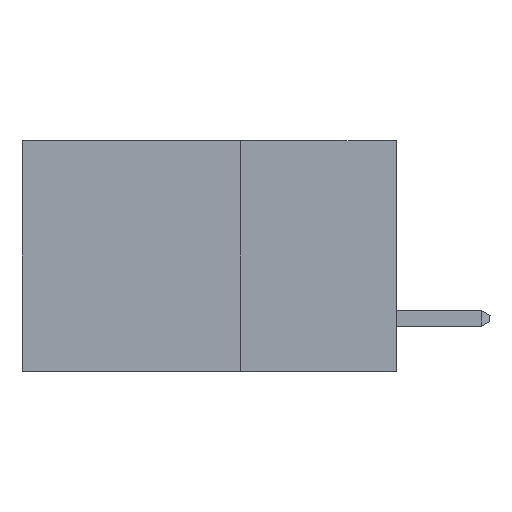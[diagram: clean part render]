
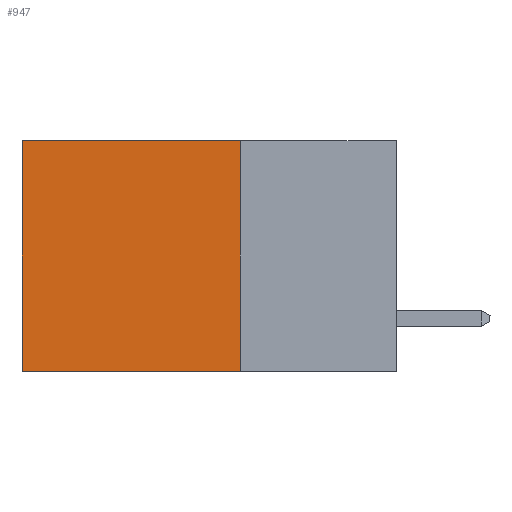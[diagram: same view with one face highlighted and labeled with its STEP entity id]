
A CAD part, left-side view. The second image highlights one B-rep face of the part: STEP entity #947.
In plain terms, the highlighted planar face has unit normal (-1, 0, 0).
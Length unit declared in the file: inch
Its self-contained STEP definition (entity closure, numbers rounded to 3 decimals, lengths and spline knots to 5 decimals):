
#130 = LINE ( 'NONE', #974, #3884 ) ;
#669 = EDGE_LOOP ( 'NONE', ( #11344, #8845, #17413, #20293 ) ) ;
#853 = FACE_OUTER_BOUND ( 'NONE', #669, .T. ) ;
#947 = ADVANCED_FACE ( 'NONE', ( #853 ), #6151, .F. ) ;
#974 = CARTESIAN_POINT ( 'NONE',  ( 0.298, 0.25, 0. ) ) ;
#1856 = VECTOR ( 'NONE', #12233, 39.37008 ) ;
#2338 = CARTESIAN_POINT ( 'NONE',  ( 0.298, 0.25, -0.37 ) ) ;
#2418 = CARTESIAN_POINT ( 'NONE',  ( 0.298, 0.25, 0. ) ) ;
#2761 = VERTEX_POINT ( 'NONE', #21534 ) ;
#3884 = VECTOR ( 'NONE', #17255, 39.37008 ) ;
#4468 = AXIS2_PLACEMENT_3D ( 'NONE', #13750, #15356, #18945 ) ;
#5245 = CARTESIAN_POINT ( 'NONE',  ( 0.298, 0.25, -0.37 ) ) ;
#6151 = PLANE ( 'NONE',  #4468 ) ;
#7152 = VECTOR ( 'NONE', #18747, 39.37008 ) ;
#8224 = LINE ( 'NONE', #8526, #1856 ) ;
#8526 = CARTESIAN_POINT ( 'NONE',  ( 0.298, 0.6, 0. ) ) ;
#8845 = ORIENTED_EDGE ( 'NONE', *, *, #14972, .F. ) ;
#11203 = LINE ( 'NONE', #18828, #7152 ) ;
#11344 = ORIENTED_EDGE ( 'NONE', *, *, #19478, .T. ) ;
#12024 = VERTEX_POINT ( 'NONE', #2418 ) ;
#12233 = DIRECTION ( 'NONE',  ( 0., 0., -1. ) ) ;
#12912 = LINE ( 'NONE', #2338, #21531 ) ;
#13750 = CARTESIAN_POINT ( 'NONE',  ( 0.298, 0.25, 0. ) ) ;
#14972 = EDGE_CURVE ( 'NONE', #23244, #2761, #12912, .T. ) ;
#15343 = DIRECTION ( 'NONE',  ( 0., 1., 0. ) ) ;
#15356 = DIRECTION ( 'NONE',  ( 1., 0., 0. ) ) ;
#16658 = CARTESIAN_POINT ( 'NONE',  ( 0.298, 0.6, 0. ) ) ;
#17255 = DIRECTION ( 'NONE',  ( 0., 0., -1. ) ) ;
#17403 = VERTEX_POINT ( 'NONE', #16658 ) ;
#17413 = ORIENTED_EDGE ( 'NONE', *, *, #19570, .F. ) ;
#17556 = EDGE_CURVE ( 'NONE', #12024, #17403, #11203, .T. ) ;
#18747 = DIRECTION ( 'NONE',  ( 0., 1., 0. ) ) ;
#18828 = CARTESIAN_POINT ( 'NONE',  ( 0.298, 0.25, 0. ) ) ;
#18945 = DIRECTION ( 'NONE',  ( 0., 0., -1. ) ) ;
#19478 = EDGE_CURVE ( 'NONE', #17403, #2761, #8224, .T. ) ;
#19570 = EDGE_CURVE ( 'NONE', #12024, #23244, #130, .T. ) ;
#20293 = ORIENTED_EDGE ( 'NONE', *, *, #17556, .T. ) ;
#21531 = VECTOR ( 'NONE', #15343, 39.37008 ) ;
#21534 = CARTESIAN_POINT ( 'NONE',  ( 0.298, 0.6, -0.37 ) ) ;
#23244 = VERTEX_POINT ( 'NONE', #5245 ) ;
